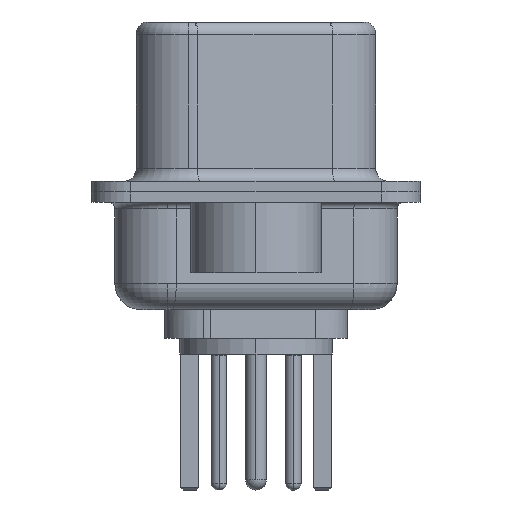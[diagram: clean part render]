
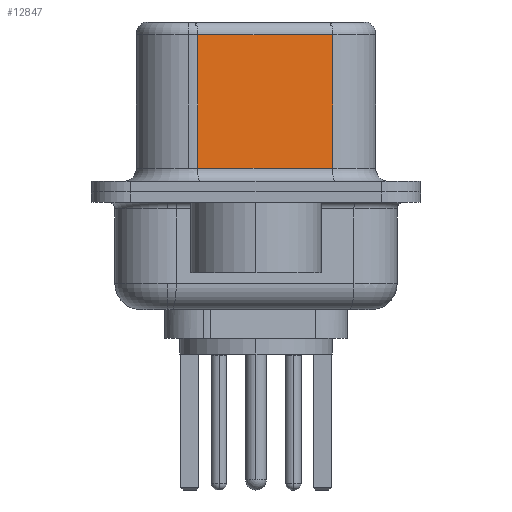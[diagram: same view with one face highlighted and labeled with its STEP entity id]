
A CAD part, left-side view. The second image highlights one B-rep face of the part: STEP entity #12847.
In plain terms, the highlighted planar face has unit normal (-0.985, -0.174, 0).
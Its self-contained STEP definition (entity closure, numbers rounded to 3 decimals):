
#870 = AXIS2_PLACEMENT_3D ( 'NONE', #17722, #19616, #7881 ) ;
#1919 = VERTEX_POINT ( 'NONE', #22334 ) ;
#2332 = ORIENTED_EDGE ( 'NONE', *, *, #23962, .T. ) ;
#3615 = VECTOR ( 'NONE', #6479, 1000. ) ;
#3840 = PLANE ( 'NONE',  #870 ) ;
#3953 = DIRECTION ( 'NONE',  ( -0.174, 0.985, 0. ) ) ;
#4480 = ORIENTED_EDGE ( 'NONE', *, *, #7326, .T. ) ;
#5171 = LINE ( 'NONE', #14820, #19589 ) ;
#5843 = CARTESIAN_POINT ( 'NONE',  ( 4.58, -2.927, 6.02 ) ) ;
#5886 = ORIENTED_EDGE ( 'NONE', *, *, #9191, .T. ) ;
#6479 = DIRECTION ( 'NONE',  ( 0., 0., -1. ) ) ;
#6519 = CARTESIAN_POINT ( 'NONE',  ( 4.58, -2.927, 6.02 ) ) ;
#6589 = CARTESIAN_POINT ( 'NONE',  ( 3.67, 2.233, 6.52 ) ) ;
#7326 = EDGE_CURVE ( 'NONE', #1919, #21537, #8553, .T. ) ;
#7881 = DIRECTION ( 'NONE',  ( -0.174, 0.985, 0. ) ) ;
#8553 = LINE ( 'NONE', #14785, #23596 ) ;
#8882 = EDGE_CURVE ( 'NONE', #13857, #21537, #5171, .T. ) ;
#9191 = EDGE_CURVE ( 'NONE', #18997, #1919, #14161, .T. ) ;
#9603 = VECTOR ( 'NONE', #3953, 1000. ) ;
#9841 = DIRECTION ( 'NONE',  ( 0.174, -0.985, 0. ) ) ;
#12847 = ADVANCED_FACE ( 'NONE', ( #16750 ), #3840, .F. ) ;
#13821 = CARTESIAN_POINT ( 'NONE',  ( 3.67, 2.233, 6.02 ) ) ;
#13857 = VERTEX_POINT ( 'NONE', #6519 ) ;
#14161 = LINE ( 'NONE', #6589, #3615 ) ;
#14785 = CARTESIAN_POINT ( 'NONE',  ( 4.58, -2.927, 0.9 ) ) ;
#14820 = CARTESIAN_POINT ( 'NONE',  ( 4.58, -2.927, 6.52 ) ) ;
#14930 = DIRECTION ( 'NONE',  ( 0., 0., -1. ) ) ;
#16750 = FACE_OUTER_BOUND ( 'NONE', #17353, .T. ) ;
#17353 = EDGE_LOOP ( 'NONE', ( #17665, #2332, #5886, #4480 ) ) ;
#17665 = ORIENTED_EDGE ( 'NONE', *, *, #8882, .F. ) ;
#17722 = CARTESIAN_POINT ( 'NONE',  ( 4.58, -2.927, 6.52 ) ) ;
#18081 = CARTESIAN_POINT ( 'NONE',  ( 4.58, -2.927, 0.9 ) ) ;
#18997 = VERTEX_POINT ( 'NONE', #13821 ) ;
#19589 = VECTOR ( 'NONE', #14930, 1000. ) ;
#19616 = DIRECTION ( 'NONE',  ( 0.985, 0.174, 0. ) ) ;
#21537 = VERTEX_POINT ( 'NONE', #18081 ) ;
#22334 = CARTESIAN_POINT ( 'NONE',  ( 3.67, 2.233, 0.9 ) ) ;
#23596 = VECTOR ( 'NONE', #9841, 1000. ) ;
#23962 = EDGE_CURVE ( 'NONE', #13857, #18997, #25307, .T. ) ;
#25307 = LINE ( 'NONE', #5843, #9603 ) ;
